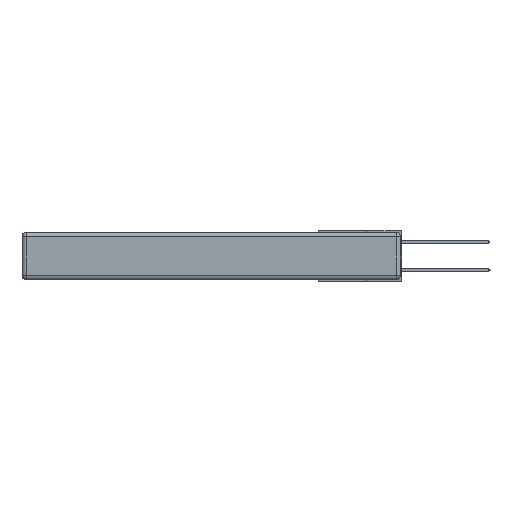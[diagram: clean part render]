
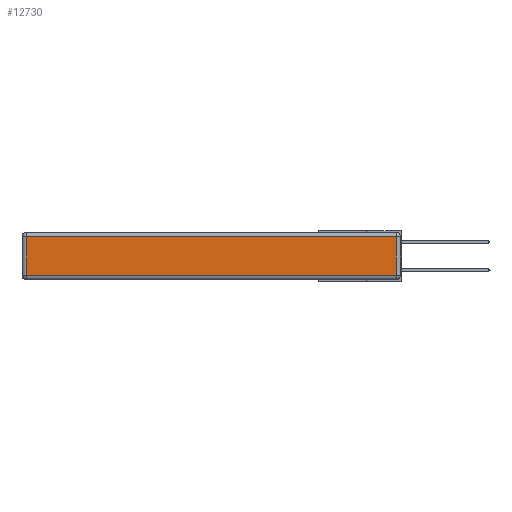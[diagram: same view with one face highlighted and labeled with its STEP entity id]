
A CAD part, left-side view. The second image highlights one B-rep face of the part: STEP entity #12730.
In plain terms, the highlighted planar face has unit normal (-1, 0, 0).
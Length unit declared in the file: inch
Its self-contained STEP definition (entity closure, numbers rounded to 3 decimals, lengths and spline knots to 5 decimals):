
#2467 = LINE ( 'NONE', #3247, #12789 ) ;
#2928 = FACE_OUTER_BOUND ( 'NONE', #7847, .T. ) ;
#3247 = CARTESIAN_POINT ( 'NONE',  ( 0., 2.75, -0.03 ) ) ;
#3425 = VERTEX_POINT ( 'NONE', #27572 ) ;
#3535 = DIRECTION ( 'NONE',  ( 0., -1., 0. ) ) ;
#4415 = CARTESIAN_POINT ( 'NONE',  ( 0., 0.03, -0.313 ) ) ;
#5747 = LINE ( 'NONE', #22150, #21076 ) ;
#6431 = EDGE_CURVE ( 'NONE', #12001, #7794, #19204, .T. ) ;
#7794 = VERTEX_POINT ( 'NONE', #9190 ) ;
#7847 = EDGE_LOOP ( 'NONE', ( #10377, #23247, #14791, #16837 ) ) ;
#8428 = EDGE_CURVE ( 'NONE', #15797, #12001, #24271, .T. ) ;
#8535 = DIRECTION ( 'NONE',  ( -1., 0., 0. ) ) ;
#9190 = CARTESIAN_POINT ( 'NONE',  ( 0., 0.03, -0.03 ) ) ;
#10275 = CARTESIAN_POINT ( 'NONE',  ( 0., 0.03, -0.343 ) ) ;
#10354 = EDGE_CURVE ( 'NONE', #7794, #3425, #2467, .T. ) ;
#10377 = ORIENTED_EDGE ( 'NONE', *, *, #8428, .T. ) ;
#11497 = DIRECTION ( 'NONE',  ( 0., 0., -1. ) ) ;
#12001 = VERTEX_POINT ( 'NONE', #4415 ) ;
#12372 = CARTESIAN_POINT ( 'NONE',  ( 0., 2.72, -0.313 ) ) ;
#12423 = DIRECTION ( 'NONE',  ( 0., 0., 1. ) ) ;
#12730 = ADVANCED_FACE ( 'NONE', ( #2928 ), #21699, .T. ) ;
#12789 = VECTOR ( 'NONE', #25428, 39.37008 ) ;
#12874 = VECTOR ( 'NONE', #12423, 39.37008 ) ;
#14791 = ORIENTED_EDGE ( 'NONE', *, *, #10354, .T. ) ;
#15797 = VERTEX_POINT ( 'NONE', #12372 ) ;
#15917 = VECTOR ( 'NONE', #3535, 39.37008 ) ;
#16837 = ORIENTED_EDGE ( 'NONE', *, *, #21530, .T. ) ;
#17272 = CARTESIAN_POINT ( 'NONE',  ( 0., 0., -0.343 ) ) ;
#19083 = AXIS2_PLACEMENT_3D ( 'NONE', #17272, #8535, #23832 ) ;
#19204 = LINE ( 'NONE', #10275, #12874 ) ;
#21076 = VECTOR ( 'NONE', #11497, 39.37008 ) ;
#21530 = EDGE_CURVE ( 'NONE', #3425, #15797, #5747, .T. ) ;
#21699 = PLANE ( 'NONE',  #19083 ) ;
#22150 = CARTESIAN_POINT ( 'NONE',  ( 0., 2.72, -0.343 ) ) ;
#23247 = ORIENTED_EDGE ( 'NONE', *, *, #6431, .T. ) ;
#23832 = DIRECTION ( 'NONE',  ( 0., 0., 1. ) ) ;
#24271 = LINE ( 'NONE', #27033, #15917 ) ;
#25428 = DIRECTION ( 'NONE',  ( 0., 1., 0. ) ) ;
#27033 = CARTESIAN_POINT ( 'NONE',  ( 0., 0., -0.313 ) ) ;
#27572 = CARTESIAN_POINT ( 'NONE',  ( 0., 2.72, -0.03 ) ) ;
